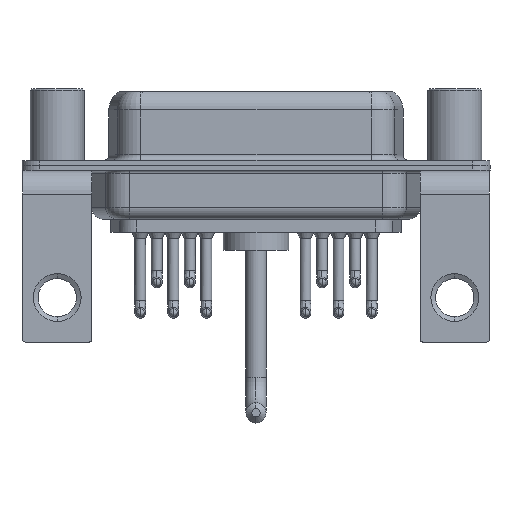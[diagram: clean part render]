
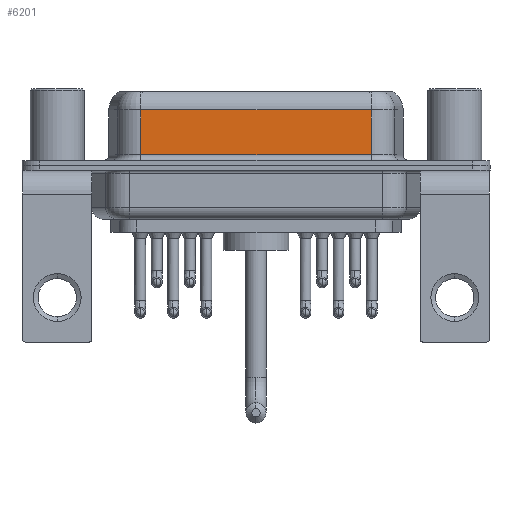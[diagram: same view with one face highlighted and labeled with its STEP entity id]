
A CAD part, front view. The second image highlights one B-rep face of the part: STEP entity #6201.
In plain terms, the highlighted planar face has unit normal (0, -1, 0).
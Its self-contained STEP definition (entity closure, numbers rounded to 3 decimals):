
#16 = VERTEX_POINT ( 'NONE', #17543 ) ;
#687 = LINE ( 'NONE', #5507, #13962 ) ;
#867 = LINE ( 'NONE', #18773, #15521 ) ;
#2465 = EDGE_CURVE ( 'NONE', #17258, #9189, #867, .T. ) ;
#3077 = ORIENTED_EDGE ( 'NONE', *, *, #13659, .T. ) ;
#3756 = LINE ( 'NONE', #15036, #4477 ) ;
#4477 = VECTOR ( 'NONE', #7295, 1000. ) ;
#5248 = EDGE_CURVE ( 'NONE', #16, #14891, #3756, .T. ) ;
#5394 = DIRECTION ( 'NONE',  ( 0., 1., 0. ) ) ;
#5507 = CARTESIAN_POINT ( 'NONE',  ( 26.287, -3.95, 4.65 ) ) ;
#6201 = ADVANCED_FACE ( 'NONE', ( #11942 ), #13451, .F. ) ;
#7295 = DIRECTION ( 'NONE',  ( 0., 0., -1. ) ) ;
#7410 = DIRECTION ( 'NONE',  ( 0., 0., -1. ) ) ;
#8517 = CARTESIAN_POINT ( 'NONE',  ( 26.287, -3.95, 4.65 ) ) ;
#9189 = VERTEX_POINT ( 'NONE', #16537 ) ;
#9266 = EDGE_CURVE ( 'NONE', #14891, #9189, #14831, .T. ) ;
#10048 = CARTESIAN_POINT ( 'NONE',  ( 7.013, -3.95, 0.9 ) ) ;
#10128 = DIRECTION ( 'NONE',  ( -1., 0., 0. ) ) ;
#11942 = FACE_OUTER_BOUND ( 'NONE', #16579, .T. ) ;
#13451 = PLANE ( 'NONE',  #14452 ) ;
#13659 = EDGE_CURVE ( 'NONE', #17258, #16, #687, .T. ) ;
#13962 = VECTOR ( 'NONE', #10128, 1000. ) ;
#14452 = AXIS2_PLACEMENT_3D ( 'NONE', #19659, #5394, #16564 ) ;
#14565 = VECTOR ( 'NONE', #19632, 1000. ) ;
#14831 = LINE ( 'NONE', #19838, #14565 ) ;
#14891 = VERTEX_POINT ( 'NONE', #10048 ) ;
#15036 = CARTESIAN_POINT ( 'NONE',  ( 7.013, -3.95, 6.4 ) ) ;
#15521 = VECTOR ( 'NONE', #7410, 1000. ) ;
#16537 = CARTESIAN_POINT ( 'NONE',  ( 26.287, -3.95, 0.9 ) ) ;
#16564 = DIRECTION ( 'NONE',  ( 0., 0., 1. ) ) ;
#16579 = EDGE_LOOP ( 'NONE', ( #17340, #3077, #18234, #20564 ) ) ;
#17258 = VERTEX_POINT ( 'NONE', #8517 ) ;
#17340 = ORIENTED_EDGE ( 'NONE', *, *, #2465, .F. ) ;
#17543 = CARTESIAN_POINT ( 'NONE',  ( 7.013, -3.95, 4.65 ) ) ;
#18234 = ORIENTED_EDGE ( 'NONE', *, *, #5248, .T. ) ;
#18773 = CARTESIAN_POINT ( 'NONE',  ( 26.287, -3.95, 6.4 ) ) ;
#19632 = DIRECTION ( 'NONE',  ( 1., 0., 0. ) ) ;
#19659 = CARTESIAN_POINT ( 'NONE',  ( 26.287, -3.95, 6.4 ) ) ;
#19838 = CARTESIAN_POINT ( 'NONE',  ( 26.287, -3.95, 0.9 ) ) ;
#20564 = ORIENTED_EDGE ( 'NONE', *, *, #9266, .T. ) ;
